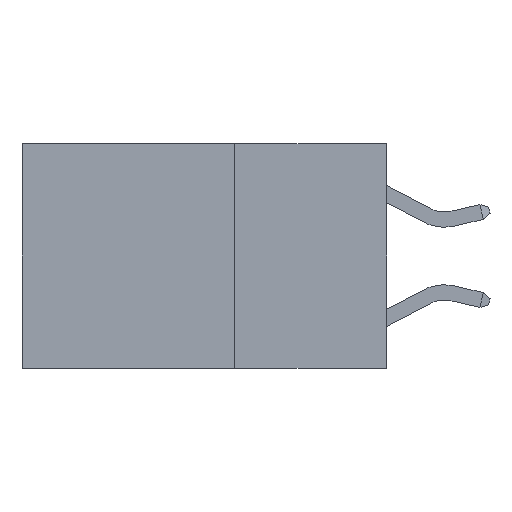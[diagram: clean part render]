
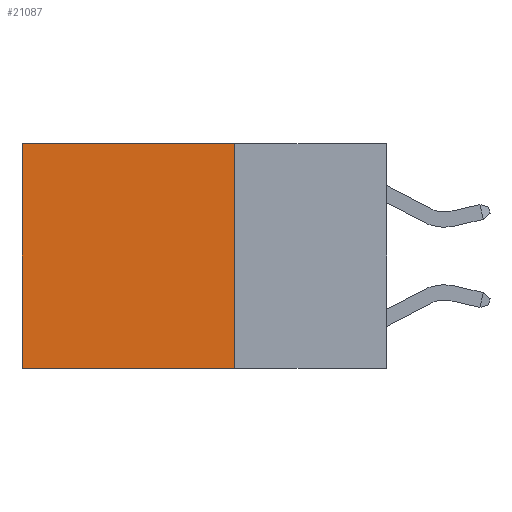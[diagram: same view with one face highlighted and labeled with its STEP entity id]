
A CAD part, left-side view. The second image highlights one B-rep face of the part: STEP entity #21087.
In plain terms, the highlighted planar face has unit normal (-1, 0, 0).
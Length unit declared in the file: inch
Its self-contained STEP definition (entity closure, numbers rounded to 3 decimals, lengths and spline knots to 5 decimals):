
#413 = CARTESIAN_POINT ( 'NONE',  ( 0.2625, 0.6, 0. ) ) ;
#2122 = VERTEX_POINT ( 'NONE', #9310 ) ;
#2433 = DIRECTION ( 'NONE',  ( 0., 0., -1. ) ) ;
#3210 = CARTESIAN_POINT ( 'NONE',  ( 0.2625, 0.6, 0. ) ) ;
#4253 = VERTEX_POINT ( 'NONE', #3210 ) ;
#4834 = ORIENTED_EDGE ( 'NONE', *, *, #19715, .T. ) ;
#6111 = CARTESIAN_POINT ( 'NONE',  ( 0.2625, 0.25, 0. ) ) ;
#7498 = LINE ( 'NONE', #9170, #9360 ) ;
#7815 = ORIENTED_EDGE ( 'NONE', *, *, #17553, .F. ) ;
#9170 = CARTESIAN_POINT ( 'NONE',  ( 0.2625, 0.25, 0. ) ) ;
#9310 = CARTESIAN_POINT ( 'NONE',  ( 0.2625, 0.6, -0.37 ) ) ;
#9313 = CARTESIAN_POINT ( 'NONE',  ( 0.2625, 0.25, 0. ) ) ;
#9360 = VECTOR ( 'NONE', #22053, 39.37008 ) ;
#10023 = DIRECTION ( 'NONE',  ( 0., 0., -1. ) ) ;
#10233 = CARTESIAN_POINT ( 'NONE',  ( 0.2625, 0.25, -0.37 ) ) ;
#10765 = ORIENTED_EDGE ( 'NONE', *, *, #14738, .F. ) ;
#11286 = VECTOR ( 'NONE', #2433, 39.37008 ) ;
#13077 = VECTOR ( 'NONE', #14278, 39.37008 ) ;
#13606 = AXIS2_PLACEMENT_3D ( 'NONE', #6111, #17644, #10023 ) ;
#13686 = ORIENTED_EDGE ( 'NONE', *, *, #17960, .T. ) ;
#14278 = DIRECTION ( 'NONE',  ( 0., 1., 0. ) ) ;
#14738 = EDGE_CURVE ( 'NONE', #15817, #2122, #16172, .T. ) ;
#15175 = FACE_OUTER_BOUND ( 'NONE', #17062, .T. ) ;
#15817 = VERTEX_POINT ( 'NONE', #18702 ) ;
#16172 = LINE ( 'NONE', #10233, #13077 ) ;
#16711 = LINE ( 'NONE', #413, #11286 ) ;
#16764 = DIRECTION ( 'NONE',  ( 0., 1., 0. ) ) ;
#17062 = EDGE_LOOP ( 'NONE', ( #4834, #10765, #7815, #13686 ) ) ;
#17553 = EDGE_CURVE ( 'NONE', #22838, #15817, #7498, .T. ) ;
#17644 = DIRECTION ( 'NONE',  ( 1., 0., 0. ) ) ;
#17960 = EDGE_CURVE ( 'NONE', #22838, #4253, #18535, .T. ) ;
#18416 = CARTESIAN_POINT ( 'NONE',  ( 0.2625, 0.25, 0. ) ) ;
#18535 = LINE ( 'NONE', #18416, #21924 ) ;
#18702 = CARTESIAN_POINT ( 'NONE',  ( 0.2625, 0.25, -0.37 ) ) ;
#19715 = EDGE_CURVE ( 'NONE', #4253, #2122, #16711, .T. ) ;
#21087 = ADVANCED_FACE ( 'NONE', ( #15175 ), #22441, .F. ) ;
#21924 = VECTOR ( 'NONE', #16764, 39.37008 ) ;
#22053 = DIRECTION ( 'NONE',  ( 0., 0., -1. ) ) ;
#22441 = PLANE ( 'NONE',  #13606 ) ;
#22838 = VERTEX_POINT ( 'NONE', #9313 ) ;
